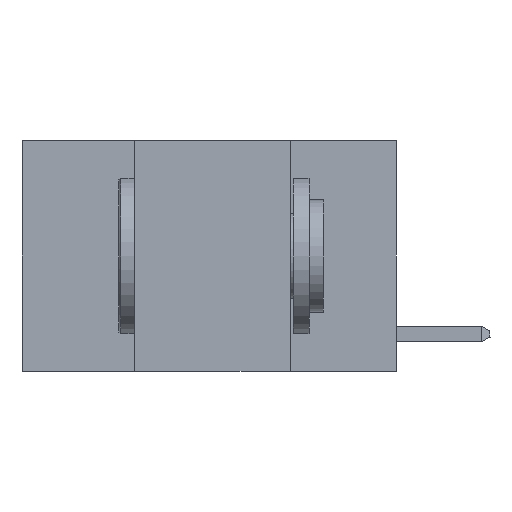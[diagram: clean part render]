
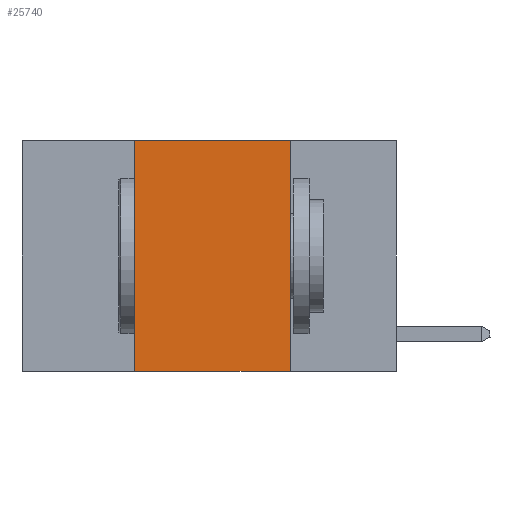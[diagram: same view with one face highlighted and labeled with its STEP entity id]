
A CAD part, left-side view. The second image highlights one B-rep face of the part: STEP entity #25740.
In plain terms, the highlighted planar face has unit normal (-1, 0, 0).
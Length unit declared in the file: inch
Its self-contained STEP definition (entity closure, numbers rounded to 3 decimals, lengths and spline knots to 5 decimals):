
#968 = CARTESIAN_POINT ( 'NONE',  ( 0., 0.6, 0. ) ) ;
#1268 = ORIENTED_EDGE ( 'NONE', *, *, #16001, .T. ) ;
#2738 = VECTOR ( 'NONE', #14973, 39.37008 ) ;
#2961 = FACE_OUTER_BOUND ( 'NONE', #25910, .T. ) ;
#3669 = VERTEX_POINT ( 'NONE', #5290 ) ;
#3954 = ORIENTED_EDGE ( 'NONE', *, *, #17139, .F. ) ;
#4148 = VECTOR ( 'NONE', #13129, 39.37008 ) ;
#4153 = VERTEX_POINT ( 'NONE', #8932 ) ;
#4516 = CARTESIAN_POINT ( 'NONE',  ( 0., 0.6, 0. ) ) ;
#5101 = DIRECTION ( 'NONE',  ( 0., -1., 0. ) ) ;
#5290 = CARTESIAN_POINT ( 'NONE',  ( 0., 0.42, -0.37 ) ) ;
#6816 = VECTOR ( 'NONE', #5101, 39.37008 ) ;
#7378 = LINE ( 'NONE', #11406, #6816 ) ;
#8932 = CARTESIAN_POINT ( 'NONE',  ( 0., 0.17, -0.37 ) ) ;
#9660 = DIRECTION ( 'NONE',  ( 0., 0., -1. ) ) ;
#10175 = CARTESIAN_POINT ( 'NONE',  ( 0., 0.17, 0. ) ) ;
#11406 = CARTESIAN_POINT ( 'NONE',  ( 0., 0.6, -0.37 ) ) ;
#12332 = EDGE_CURVE ( 'NONE', #18477, #4153, #27685, .T. ) ;
#13129 = DIRECTION ( 'NONE',  ( 0., 0., 1. ) ) ;
#14866 = LINE ( 'NONE', #23624, #4148 ) ;
#14973 = DIRECTION ( 'NONE',  ( 0., -1., 0. ) ) ;
#15115 = LINE ( 'NONE', #4516, #2738 ) ;
#15761 = ORIENTED_EDGE ( 'NONE', *, *, #16267, .F. ) ;
#16001 = EDGE_CURVE ( 'NONE', #3669, #4153, #7378, .T. ) ;
#16267 = EDGE_CURVE ( 'NONE', #26515, #18477, #15115, .T. ) ;
#17139 = EDGE_CURVE ( 'NONE', #3669, #26515, #14866, .T. ) ;
#17416 = AXIS2_PLACEMENT_3D ( 'NONE', #968, #17854, #9660 ) ;
#17854 = DIRECTION ( 'NONE',  ( 1., 0., 0. ) ) ;
#18285 = PLANE ( 'NONE',  #17416 ) ;
#18477 = VERTEX_POINT ( 'NONE', #10175 ) ;
#20967 = DIRECTION ( 'NONE',  ( 0., 0., -1. ) ) ;
#21158 = ORIENTED_EDGE ( 'NONE', *, *, #12332, .F. ) ;
#21534 = CARTESIAN_POINT ( 'NONE',  ( 0., 0.17, 0. ) ) ;
#23609 = CARTESIAN_POINT ( 'NONE',  ( 0., 0.42, 0. ) ) ;
#23624 = CARTESIAN_POINT ( 'NONE',  ( 0., 0.42, 0. ) ) ;
#23661 = VECTOR ( 'NONE', #20967, 39.37008 ) ;
#25740 = ADVANCED_FACE ( 'NONE', ( #2961 ), #18285, .F. ) ;
#25910 = EDGE_LOOP ( 'NONE', ( #21158, #15761, #3954, #1268 ) ) ;
#26515 = VERTEX_POINT ( 'NONE', #23609 ) ;
#27685 = LINE ( 'NONE', #21534, #23661 ) ;
